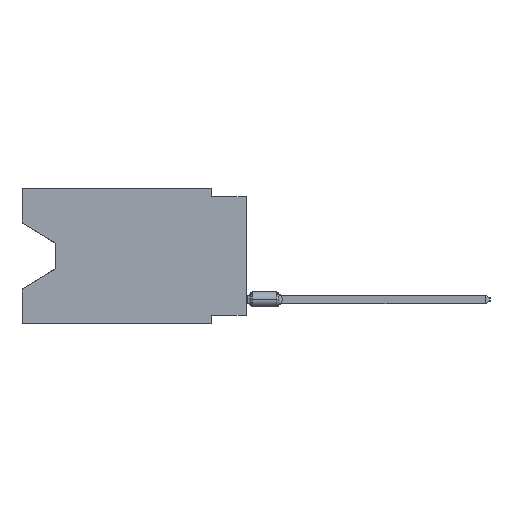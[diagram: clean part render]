
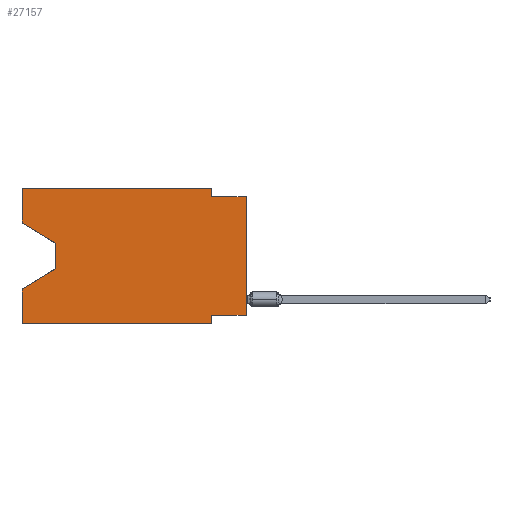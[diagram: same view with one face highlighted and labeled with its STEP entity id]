
A CAD part, left-side view. The second image highlights one B-rep face of the part: STEP entity #27157.
In plain terms, the highlighted planar face has unit normal (-1, 0, 0).
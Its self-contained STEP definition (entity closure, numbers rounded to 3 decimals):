
#272 = VECTOR ( 'NONE', #75162, 1000. ) ;
#901 = ORIENTED_EDGE ( 'NONE', *, *, #25591, .T. ) ;
#3052 = EDGE_CURVE ( 'NONE', #70545, #63946, #8129, .T. ) ;
#4012 = VERTEX_POINT ( 'NONE', #37433 ) ;
#4723 = CARTESIAN_POINT ( 'NONE',  ( 0., 0., -9.271 ) ) ;
#5827 = ORIENTED_EDGE ( 'NONE', *, *, #44477, .T. ) ;
#6420 = CARTESIAN_POINT ( 'NONE',  ( 0., 16.383, 0. ) ) ;
#8097 = CARTESIAN_POINT ( 'NONE',  ( 0., 0., 0. ) ) ;
#8129 = LINE ( 'NONE', #57805, #44669 ) ;
#8574 = EDGE_CURVE ( 'NONE', #28770, #9735, #60297, .T. ) ;
#9061 = VECTOR ( 'NONE', #61429, 1000. ) ;
#9331 = VERTEX_POINT ( 'NONE', #39117 ) ;
#9735 = VERTEX_POINT ( 'NONE', #33370 ) ;
#9876 = EDGE_CURVE ( 'NONE', #35650, #70435, #13399, .T. ) ;
#10370 = VECTOR ( 'NONE', #29592, 1000. ) ;
#11753 = VECTOR ( 'NONE', #18266, 1000. ) ;
#12096 = DIRECTION ( 'NONE',  ( 0., -0.855, -0.519 ) ) ;
#12218 = CARTESIAN_POINT ( 'NONE',  ( 0., 13.97, -5.893 ) ) ;
#12877 = LINE ( 'NONE', #6420, #13971 ) ;
#13101 = ORIENTED_EDGE ( 'NONE', *, *, #37756, .F. ) ;
#13103 = DIRECTION ( 'NONE',  ( 0., 0., -1. ) ) ;
#13399 = LINE ( 'NONE', #55446, #11753 ) ;
#13971 = VECTOR ( 'NONE', #44748, 1000. ) ;
#14158 = DIRECTION ( 'NONE',  ( 1., 0., 0. ) ) ;
#14159 = LINE ( 'NONE', #8097, #272 ) ;
#14881 = ORIENTED_EDGE ( 'NONE', *, *, #32138, .F. ) ;
#16043 = ORIENTED_EDGE ( 'NONE', *, *, #55669, .F. ) ;
#16904 = VECTOR ( 'NONE', #19411, 1000. ) ;
#17872 = ORIENTED_EDGE ( 'NONE', *, *, #8574, .F. ) ;
#18266 = DIRECTION ( 'NONE',  ( 0., 0.855, -0.519 ) ) ;
#18568 = VERTEX_POINT ( 'NONE', #41383 ) ;
#19411 = DIRECTION ( 'NONE',  ( 0., 0., -1. ) ) ;
#20992 = PLANE ( 'NONE',  #73674 ) ;
#21610 = CARTESIAN_POINT ( 'NONE',  ( 0., 16.383, -9.906 ) ) ;
#22510 = VECTOR ( 'NONE', #75700, 1000. ) ;
#24250 = LINE ( 'NONE', #54178, #9061 ) ;
#25321 = ORIENTED_EDGE ( 'NONE', *, *, #63196, .F. ) ;
#25591 = EDGE_CURVE ( 'NONE', #18568, #67661, #54914, .T. ) ;
#25877 = CARTESIAN_POINT ( 'NONE',  ( 0., 2.54, 0. ) ) ;
#27090 = EDGE_CURVE ( 'NONE', #4012, #28770, #74777, .T. ) ;
#27157 = ADVANCED_FACE ( 'NONE', ( #70683 ), #20992, .F. ) ;
#28724 = LINE ( 'NONE', #54559, #79543 ) ;
#28770 = VERTEX_POINT ( 'NONE', #52016 ) ;
#29592 = DIRECTION ( 'NONE',  ( 0., -1., 0. ) ) ;
#32138 = EDGE_CURVE ( 'NONE', #77526, #70435, #63190, .T. ) ;
#32337 = CARTESIAN_POINT ( 'NONE',  ( 0., 16.383, 0. ) ) ;
#33126 = DIRECTION ( 'NONE',  ( 0., 0., -1. ) ) ;
#33370 = CARTESIAN_POINT ( 'NONE',  ( 0., 0., -0.635 ) ) ;
#33504 = CARTESIAN_POINT ( 'NONE',  ( 0., 2.54, -9.271 ) ) ;
#35650 = VERTEX_POINT ( 'NONE', #12218 ) ;
#36523 = VERTEX_POINT ( 'NONE', #45400 ) ;
#37433 = CARTESIAN_POINT ( 'NONE',  ( 0., 2.54, 0. ) ) ;
#37756 = EDGE_CURVE ( 'NONE', #9331, #4012, #12877, .T. ) ;
#38366 = CARTESIAN_POINT ( 'NONE',  ( 0., 13.97, -4.013 ) ) ;
#39117 = CARTESIAN_POINT ( 'NONE',  ( 0., 16.383, 0. ) ) ;
#39851 = EDGE_CURVE ( 'NONE', #67661, #35650, #68455, .T. ) ;
#41216 = CARTESIAN_POINT ( 'NONE',  ( 0., 16.383, -2.546 ) ) ;
#41383 = CARTESIAN_POINT ( 'NONE',  ( 0., 16.383, -2.546 ) ) ;
#44477 = EDGE_CURVE ( 'NONE', #77526, #36523, #49670, .T. ) ;
#44669 = VECTOR ( 'NONE', #70314, 1000. ) ;
#44748 = DIRECTION ( 'NONE',  ( 0., -1., 0. ) ) ;
#45400 = CARTESIAN_POINT ( 'NONE',  ( 0., 2.54, -9.906 ) ) ;
#47708 = DIRECTION ( 'NONE',  ( 0., 0., 1. ) ) ;
#49670 = LINE ( 'NONE', #75116, #78662 ) ;
#52016 = CARTESIAN_POINT ( 'NONE',  ( 0., 2.54, -0.635 ) ) ;
#54178 = CARTESIAN_POINT ( 'NONE',  ( 0., 2.54, -9.906 ) ) ;
#54559 = CARTESIAN_POINT ( 'NONE',  ( 0., 16.383, 0. ) ) ;
#54914 = LINE ( 'NONE', #41216, #69622 ) ;
#55446 = CARTESIAN_POINT ( 'NONE',  ( 0., 13.97, -5.893 ) ) ;
#55669 = EDGE_CURVE ( 'NONE', #63946, #36523, #24250, .T. ) ;
#56727 = CARTESIAN_POINT ( 'NONE',  ( 0., 16.383, 0. ) ) ;
#56933 = DIRECTION ( 'NONE',  ( 0., -1., 0. ) ) ;
#57119 = CARTESIAN_POINT ( 'NONE',  ( 0., 13.97, -4.013 ) ) ;
#57675 = CARTESIAN_POINT ( 'NONE',  ( 0., 16.383, -7.36 ) ) ;
#57740 = EDGE_CURVE ( 'NONE', #70545, #9735, #14159, .T. ) ;
#57805 = CARTESIAN_POINT ( 'NONE',  ( 0., 0., -9.271 ) ) ;
#59381 = ORIENTED_EDGE ( 'NONE', *, *, #39851, .T. ) ;
#59507 = CARTESIAN_POINT ( 'NONE',  ( 0., 0., -0.635 ) ) ;
#60297 = LINE ( 'NONE', #59507, #10370 ) ;
#61429 = DIRECTION ( 'NONE',  ( 0., 0., -1. ) ) ;
#63190 = LINE ( 'NONE', #56727, #22510 ) ;
#63196 = EDGE_CURVE ( 'NONE', #18568, #9331, #28724, .T. ) ;
#63548 = ORIENTED_EDGE ( 'NONE', *, *, #27090, .F. ) ;
#63946 = VERTEX_POINT ( 'NONE', #33504 ) ;
#67661 = VERTEX_POINT ( 'NONE', #38366 ) ;
#68455 = LINE ( 'NONE', #57119, #71666 ) ;
#69353 = ORIENTED_EDGE ( 'NONE', *, *, #9876, .T. ) ;
#69622 = VECTOR ( 'NONE', #12096, 1000. ) ;
#70314 = DIRECTION ( 'NONE',  ( 0., 1., 0. ) ) ;
#70435 = VERTEX_POINT ( 'NONE', #57675 ) ;
#70545 = VERTEX_POINT ( 'NONE', #4723 ) ;
#70683 = FACE_OUTER_BOUND ( 'NONE', #78797, .T. ) ;
#71666 = VECTOR ( 'NONE', #13103, 1000. ) ;
#73674 = AXIS2_PLACEMENT_3D ( 'NONE', #32337, #14158, #33126 ) ;
#74638 = ORIENTED_EDGE ( 'NONE', *, *, #57740, .T. ) ;
#74777 = LINE ( 'NONE', #25877, #16904 ) ;
#75114 = ORIENTED_EDGE ( 'NONE', *, *, #3052, .F. ) ;
#75116 = CARTESIAN_POINT ( 'NONE',  ( 0., 16.383, -9.906 ) ) ;
#75162 = DIRECTION ( 'NONE',  ( 0., 0., 1. ) ) ;
#75700 = DIRECTION ( 'NONE',  ( 0., 0., 1. ) ) ;
#77526 = VERTEX_POINT ( 'NONE', #21610 ) ;
#78662 = VECTOR ( 'NONE', #56933, 1000. ) ;
#78797 = EDGE_LOOP ( 'NONE', ( #901, #59381, #69353, #14881, #5827, #16043, #75114, #74638, #17872, #63548, #13101, #25321 ) ) ;
#79543 = VECTOR ( 'NONE', #47708, 1000. ) ;
